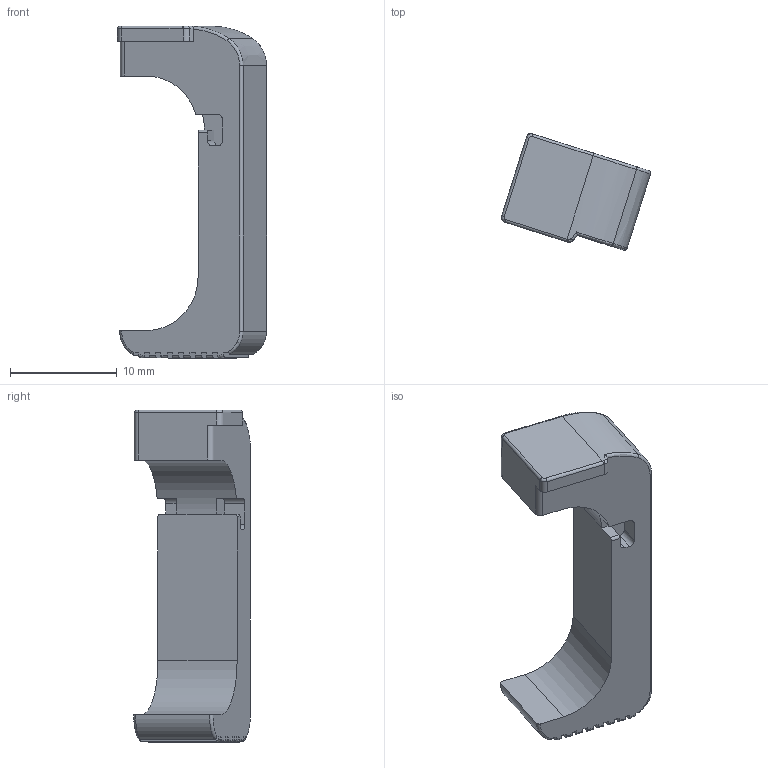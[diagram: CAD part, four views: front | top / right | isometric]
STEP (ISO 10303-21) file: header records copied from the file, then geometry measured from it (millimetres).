
FILE_DESCRIPTION(/* description */ (''),/* implementation_level */ '2;1');
FILE_NAME(/* name */ 'PrintYour2A Gen5 Mag Release 6.0.step',/* time_stamp */ '2021-10-31T15:38:52-04:00',/* author */ (''),/* organization */ (''),/* preprocessor_version */ 'ST-DEVELOPER v18.1',/* originating_system */ 'Autodesk Translation Framework v10.10.0.1391',/* authorisation */ '');
FILE_SCHEMA (('AUTOMOTIVE_DESIGN { 1 0 10303 214 3 1 1 }'));
Length unit declared in the file: millimetre
Products named in the file (1): PY2A G34 Gen5
Bounding box: 13.96 x 10.93 x 31.11 mm (x, y, z)
Volume: 1488.3 mm3; surface area: 1206.2 mm2
Topology: 1 solids, 1 shells, 110 faces, 309 edges, 201 vertices
Faces by surface type: plane 56, cylinder 35, bspline 11, torus 8
Entity records: 3896 total; most frequent: CARTESIAN_POINT 1053, ORIENTED_EDGE 620, DIRECTION 562, EDGE_CURVE 310, VERTEX_POINT 202, LINE 188, VECTOR 188, AXIS2_PLACEMENT_3D 187
